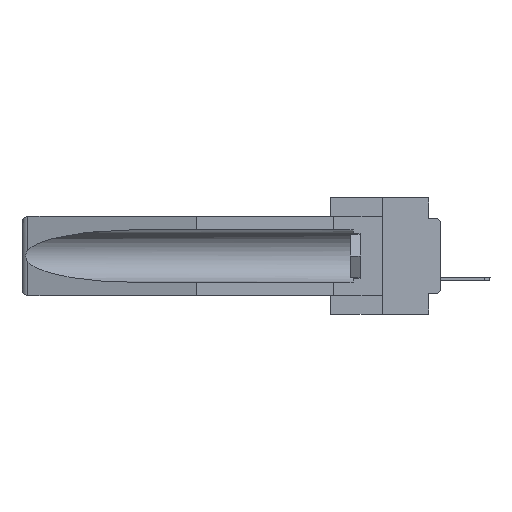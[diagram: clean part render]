
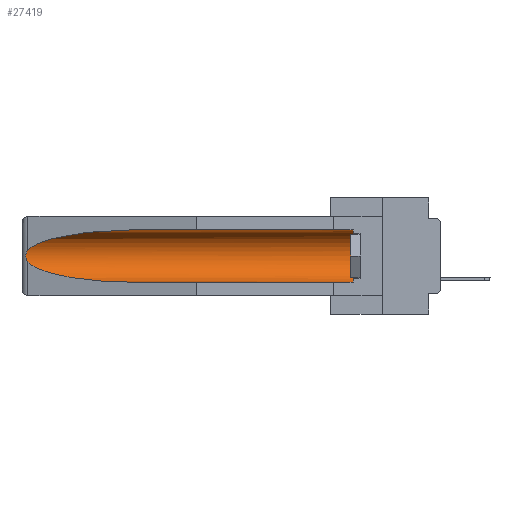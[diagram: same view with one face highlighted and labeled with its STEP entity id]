
A CAD part, left-side view. The second image highlights one B-rep face of the part: STEP entity #27419.
In plain terms, the highlighted cylindrical face has radius 2.857 mm (diameter 5.715 mm), a partial arc.
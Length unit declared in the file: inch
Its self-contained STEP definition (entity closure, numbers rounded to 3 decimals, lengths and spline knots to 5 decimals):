
#1934 = VERTEX_POINT ( 'NONE', #11341 ) ;
#2256 = CARTESIAN_POINT ( 'NONE',  ( 0.25451, 1.48313, -0.24835 ) ) ;
#2899 = LINE ( 'NONE', #29763, #34412 ) ;
#3006 = B_SPLINE_CURVE_WITH_KNOTS ( 'NONE', 3,
 ( #22000, #24582, #16507, #16281, #13586, #11003, #36168, #8119, #13704, #30274 ),
 .UNSPECIFIED., .F., .F.,
 ( 4, 2, 2, 2, 4 ),
 ( 0., 0.00029, 0.00058, 0.00087, 0.00117 ),
 .UNSPECIFIED. ) ;
#3097 = CARTESIAN_POINT ( 'NONE',  ( 0.21114, 1.30732, -0.059 ) ) ;
#3211 = EDGE_CURVE ( 'NONE', #25494, #6237, #2899, .T. ) ;
#3441 = CARTESIAN_POINT ( 'NONE',  ( 0.25451, 1.48313, -0.09465 ) ) ;
#4374 = EDGE_CURVE ( 'NONE', #25494, #13233, #32166, .T. ) ;
#5539 = ORIENTED_EDGE ( 'NONE', *, *, #19531, .T. ) ;
#5625 = ORIENTED_EDGE ( 'NONE', *, *, #4374, .T. ) ;
#6124 = CARTESIAN_POINT ( 'NONE',  ( 0.155, -0.30754, -0.059 ) ) ;
#6237 = VERTEX_POINT ( 'NONE', #21216 ) ;
#6333 = CYLINDRICAL_SURFACE ( 'NONE', #33265, 0.1125 ) ;
#7104 = CARTESIAN_POINT ( 'NONE',  ( 0.26537, 1.52718, -0.19328 ) ) ;
#8119 = CARTESIAN_POINT ( 'NONE',  ( 0.26655, 1.53094, -0.18657 ) ) ;
#8662 = CARTESIAN_POINT ( 'NONE',  ( 0.155, 1.07973, -0.059 ) ) ;
#11003 = CARTESIAN_POINT ( 'NONE',  ( 0.2675, 1.53308, -0.17534 ) ) ;
#11341 = CARTESIAN_POINT ( 'NONE',  ( 0.26537, 1.52718, -0.14972 ) ) ;
#11907 = ORIENTED_EDGE ( 'NONE', *, *, #34389, .T. ) ;
#12243 = DIRECTION ( 'NONE',  ( 0., -1., 0. ) ) ;
#12372 = VERTEX_POINT ( 'NONE', #31436 ) ;
#12976 = CARTESIAN_POINT ( 'NONE',  ( 0.155, 0.126, -0.059 ) ) ;
#13233 = VERTEX_POINT ( 'NONE', #12976 ) ;
#13398 =( BOUNDED_CURVE ( )  B_SPLINE_CURVE ( 3, ( #8662, #3097, #3441, #23012 ),
 .UNSPECIFIED., .F., .F. ) 
 B_SPLINE_CURVE_WITH_KNOTS ( ( 4, 4 ),
 ( 4.71239, 6.08839 ),
 .UNSPECIFIED. ) 
 CURVE ( )  GEOMETRIC_REPRESENTATION_ITEM ( )  RATIONAL_B_SPLINE_CURVE ( ( 1., 0.848, 0.848, 1. ) ) 
 REPRESENTATION_ITEM ( '' )  );
#13586 = CARTESIAN_POINT ( 'NONE',  ( 0.2675, 1.53308, -0.16763 ) ) ;
#13704 = CARTESIAN_POINT ( 'NONE',  ( 0.26597, 1.5296, -0.19026 ) ) ;
#13744 = CARTESIAN_POINT ( 'NONE',  ( 0.21114, 1.30732, -0.284 ) ) ;
#14538 = DIRECTION ( 'NONE',  ( 0., 1., 0. ) ) ;
#16281 = CARTESIAN_POINT ( 'NONE',  ( 0.2673, 1.5327, -0.16383 ) ) ;
#16507 = CARTESIAN_POINT ( 'NONE',  ( 0.26654, 1.53092, -0.15636 ) ) ;
#17851 = DIRECTION ( 'NONE',  ( 0., 0., 1. ) ) ;
#18196 = FACE_OUTER_BOUND ( 'NONE', #19757, .T. ) ;
#19251 = CARTESIAN_POINT ( 'NONE',  ( 0.155, 1.07973, -0.284 ) ) ;
#19531 = EDGE_CURVE ( 'NONE', #12372, #1934, #13398, .T. ) ;
#19757 = EDGE_LOOP ( 'NONE', ( #5539, #11907, #35220, #31296, #5625, #19999 ) ) ;
#19999 = ORIENTED_EDGE ( 'NONE', *, *, #24024, .T. ) ;
#20054 = CARTESIAN_POINT ( 'NONE',  ( 0.155, -0.30754, -0.1715 ) ) ;
#21110 = VECTOR ( 'NONE', #31254, 39.37008 ) ;
#21216 = CARTESIAN_POINT ( 'NONE',  ( 0.155, 1.07973, -0.284 ) ) ;
#22000 = CARTESIAN_POINT ( 'NONE',  ( 0.26537, 1.52718, -0.14972 ) ) ;
#23012 = CARTESIAN_POINT ( 'NONE',  ( 0.26537, 1.52718, -0.14972 ) ) ;
#24024 = EDGE_CURVE ( 'NONE', #13233, #12372, #28481, .T. ) ;
#24582 = CARTESIAN_POINT ( 'NONE',  ( 0.26597, 1.52961, -0.15275 ) ) ;
#25494 = VERTEX_POINT ( 'NONE', #27297 ) ;
#27102 = DIRECTION ( 'NONE',  ( 0., 1., 0. ) ) ;
#27297 = CARTESIAN_POINT ( 'NONE',  ( 0.155, 0.126, -0.284 ) ) ;
#27419 = ADVANCED_FACE ( 'NONE', ( #18196 ), #6333, .F. ) ;
#27646 = CARTESIAN_POINT ( 'NONE',  ( 0.26537, 1.52718, -0.19328 ) ) ;
#28481 = LINE ( 'NONE', #6124, #21110 ) ;
#29763 = CARTESIAN_POINT ( 'NONE',  ( 0.155, -0.30754, -0.284 ) ) ;
#30274 = CARTESIAN_POINT ( 'NONE',  ( 0.26537, 1.52718, -0.19328 ) ) ;
#30640 = VERTEX_POINT ( 'NONE', #7104 ) ;
#31254 = DIRECTION ( 'NONE',  ( 0., 1., 0. ) ) ;
#31296 = ORIENTED_EDGE ( 'NONE', *, *, #3211, .F. ) ;
#31436 = CARTESIAN_POINT ( 'NONE',  ( 0.155, 1.07973, -0.059 ) ) ;
#31533 = EDGE_CURVE ( 'NONE', #30640, #6237, #31733, .T. ) ;
#31733 =( BOUNDED_CURVE ( )  B_SPLINE_CURVE ( 3, ( #27646, #2256, #13744, #19251 ),
 .UNSPECIFIED., .F., .F. ) 
 B_SPLINE_CURVE_WITH_KNOTS ( ( 4, 4 ),
 ( 0.1948, 1.5708 ),
 .UNSPECIFIED. ) 
 CURVE ( )  GEOMETRIC_REPRESENTATION_ITEM ( )  RATIONAL_B_SPLINE_CURVE ( ( 1., 0.848, 0.848, 1. ) ) 
 REPRESENTATION_ITEM ( '' )  );
#32027 = CARTESIAN_POINT ( 'NONE',  ( 0.155, 0.126, -0.1715 ) ) ;
#32166 = CIRCLE ( 'NONE', #32483, 0.1125 ) ;
#32483 = AXIS2_PLACEMENT_3D ( 'NONE', #32027, #12243, #17851 ) ;
#33265 = AXIS2_PLACEMENT_3D ( 'NONE', #20054, #14538, #34073 ) ;
#34073 = DIRECTION ( 'NONE',  ( 0., 0., 1. ) ) ;
#34389 = EDGE_CURVE ( 'NONE', #1934, #30640, #3006, .T. ) ;
#34412 = VECTOR ( 'NONE', #27102, 39.37008 ) ;
#35220 = ORIENTED_EDGE ( 'NONE', *, *, #31533, .T. ) ;
#36168 = CARTESIAN_POINT ( 'NONE',  ( 0.2673, 1.53269, -0.17917 ) ) ;
